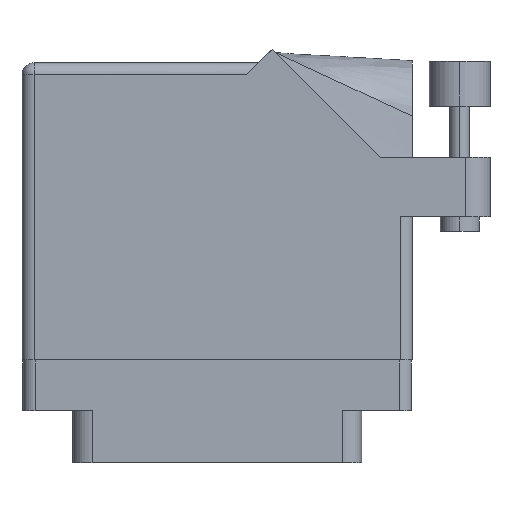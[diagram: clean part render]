
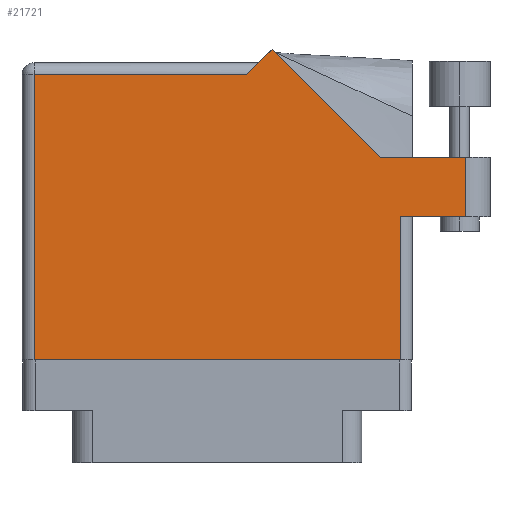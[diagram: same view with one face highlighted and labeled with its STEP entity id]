
A CAD part, front view. The second image highlights one B-rep face of the part: STEP entity #21721.
In plain terms, the highlighted face is planar.
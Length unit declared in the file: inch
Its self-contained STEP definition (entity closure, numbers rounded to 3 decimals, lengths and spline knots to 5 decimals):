
#8 = VECTOR ( 'NONE', #28993, 39.37008 ) ;
#1436 = LINE ( 'NONE', #5551, #14909 ) ;
#1519 = DIRECTION ( 'NONE',  ( -0.707, -0.707, 0. ) ) ;
#1725 = LINE ( 'NONE', #20734, #8 ) ;
#2621 = VERTEX_POINT ( 'NONE', #11171 ) ;
#4352 = EDGE_CURVE ( 'NONE', #29383, #14098, #9765, .T. ) ;
#4702 = VECTOR ( 'NONE', #5446, 39.37008 ) ;
#5280 = VECTOR ( 'NONE', #1519, 39.37008 ) ;
#5446 = DIRECTION ( 'NONE',  ( 0., -1., 0. ) ) ;
#5458 = EDGE_LOOP ( 'NONE', ( #15578, #28606, #12613, #14121, #14128, #9801, #17689, #9882, #34593 ) ) ;
#5551 = CARTESIAN_POINT ( 'NONE',  ( 1.84442, 1.044, 0. ) ) ;
#6609 = CARTESIAN_POINT ( 'NONE',  ( 0.062, 1.468, 0. ) ) ;
#6765 = VECTOR ( 'NONE', #17985, 39.37008 ) ;
#7063 = VECTOR ( 'NONE', #13210, 39.37008 ) ;
#7862 = AXIS2_PLACEMENT_3D ( 'NONE', #27327, #11181, #30057 ) ;
#7960 = CARTESIAN_POINT ( 'NONE',  ( 1.28771, 1.60071, 0. ) ) ;
#8096 = CARTESIAN_POINT ( 'NONE',  ( 0.062, 0., 0. ) ) ;
#9168 = LINE ( 'NONE', #13095, #7063 ) ;
#9765 = LINE ( 'NONE', #14557, #23250 ) ;
#9801 = ORIENTED_EDGE ( 'NONE', *, *, #23828, .T. ) ;
#9882 = ORIENTED_EDGE ( 'NONE', *, *, #12188, .T. ) ;
#10731 = LINE ( 'NONE', #17966, #5280 ) ;
#11171 = CARTESIAN_POINT ( 'NONE',  ( 1.155, 1.468, 0. ) ) ;
#11181 = DIRECTION ( 'NONE',  ( 0., 0., -1. ) ) ;
#11562 = FACE_OUTER_BOUND ( 'NONE', #5458, .T. ) ;
#12188 = EDGE_CURVE ( 'NONE', #19572, #31687, #17808, .T. ) ;
#12613 = ORIENTED_EDGE ( 'NONE', *, *, #4352, .T. ) ;
#13095 = CARTESIAN_POINT ( 'NONE',  ( 2.01, 0.737, 0. ) ) ;
#13210 = DIRECTION ( 'NONE',  ( 1., 0., 0. ) ) ;
#13617 = EDGE_CURVE ( 'NONE', #30850, #29383, #1725, .T. ) ;
#14098 = VERTEX_POINT ( 'NONE', #15830 ) ;
#14121 = ORIENTED_EDGE ( 'NONE', *, *, #18218, .T. ) ;
#14128 = ORIENTED_EDGE ( 'NONE', *, *, #25057, .T. ) ;
#14131 = VECTOR ( 'NONE', #18329, 39.37008 ) ;
#14557 = CARTESIAN_POINT ( 'NONE',  ( 2.41, 1.044, 0. ) ) ;
#14909 = VECTOR ( 'NONE', #32874, 39.37008 ) ;
#15578 = ORIENTED_EDGE ( 'NONE', *, *, #29676, .T. ) ;
#15830 = CARTESIAN_POINT ( 'NONE',  ( 1.84442, 1.044, 0. ) ) ;
#17689 = ORIENTED_EDGE ( 'NONE', *, *, #19021, .T. ) ;
#17808 = LINE ( 'NONE', #25164, #23264 ) ;
#17966 = CARTESIAN_POINT ( 'NONE',  ( 1.217, 1.53, 0. ) ) ;
#17985 = DIRECTION ( 'NONE',  ( 0., 1., 0. ) ) ;
#18218 = EDGE_CURVE ( 'NONE', #14098, #26891, #1436, .T. ) ;
#18329 = DIRECTION ( 'NONE',  ( -1., 0., 0. ) ) ;
#19021 = EDGE_CURVE ( 'NONE', #27162, #19572, #22413, .T. ) ;
#19572 = VERTEX_POINT ( 'NONE', #23420 ) ;
#19749 = DIRECTION ( 'NONE',  ( 1., 0., 0. ) ) ;
#20400 = CARTESIAN_POINT ( 'NONE',  ( 2.285, 1.044, 0. ) ) ;
#20734 = CARTESIAN_POINT ( 'NONE',  ( 2.285, 1.044, 0. ) ) ;
#21721 = ADVANCED_FACE ( 'NONE', ( #11562 ), #27441, .F. ) ;
#22318 = DIRECTION ( 'NONE',  ( -1., 0., 0. ) ) ;
#22413 = LINE ( 'NONE', #8096, #4702 ) ;
#22596 = CARTESIAN_POINT ( 'NONE',  ( 1.948, 0.737, 0. ) ) ;
#23250 = VECTOR ( 'NONE', #22318, 39.37008 ) ;
#23264 = VECTOR ( 'NONE', #19749, 39.37008 ) ;
#23420 = CARTESIAN_POINT ( 'NONE',  ( 0.062, 0., 0. ) ) ;
#23828 = EDGE_CURVE ( 'NONE', #2621, #27162, #29319, .T. ) ;
#25057 = EDGE_CURVE ( 'NONE', #26891, #2621, #10731, .T. ) ;
#25164 = CARTESIAN_POINT ( 'NONE',  ( 0., 0., 0. ) ) ;
#26891 = VERTEX_POINT ( 'NONE', #7960 ) ;
#27007 = CARTESIAN_POINT ( 'NONE',  ( 1.948, 0., 0. ) ) ;
#27162 = VERTEX_POINT ( 'NONE', #6609 ) ;
#27327 = CARTESIAN_POINT ( 'NONE',  ( 0., 1.53, 0. ) ) ;
#27441 = PLANE ( 'NONE',  #7862 ) ;
#28606 = ORIENTED_EDGE ( 'NONE', *, *, #13617, .T. ) ;
#28698 = LINE ( 'NONE', #30523, #6765 ) ;
#28993 = DIRECTION ( 'NONE',  ( 0., 1., 0. ) ) ;
#29173 = CARTESIAN_POINT ( 'NONE',  ( 0., 1.468, 0. ) ) ;
#29319 = LINE ( 'NONE', #29173, #14131 ) ;
#29383 = VERTEX_POINT ( 'NONE', #20400 ) ;
#29676 = EDGE_CURVE ( 'NONE', #31198, #30850, #9168, .T. ) ;
#30057 = DIRECTION ( 'NONE',  ( -1., 0., 0. ) ) ;
#30523 = CARTESIAN_POINT ( 'NONE',  ( 1.948, 0.737, 0. ) ) ;
#30850 = VERTEX_POINT ( 'NONE', #32916 ) ;
#31198 = VERTEX_POINT ( 'NONE', #22596 ) ;
#31687 = VERTEX_POINT ( 'NONE', #27007 ) ;
#32874 = DIRECTION ( 'NONE',  ( -0.707, 0.707, 0. ) ) ;
#32916 = CARTESIAN_POINT ( 'NONE',  ( 2.285, 0.737, 0. ) ) ;
#33737 = EDGE_CURVE ( 'NONE', #31687, #31198, #28698, .T. ) ;
#34593 = ORIENTED_EDGE ( 'NONE', *, *, #33737, .T. ) ;
